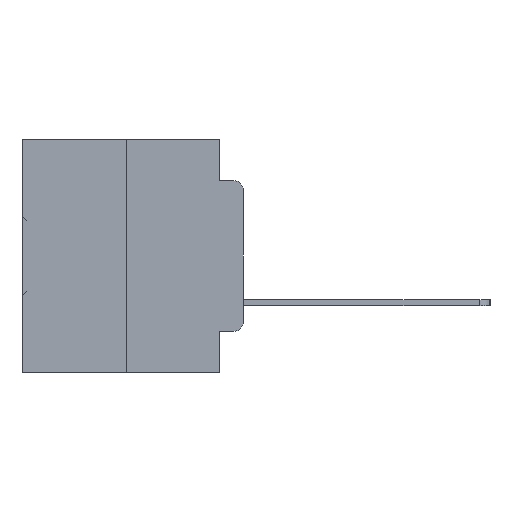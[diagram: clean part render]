
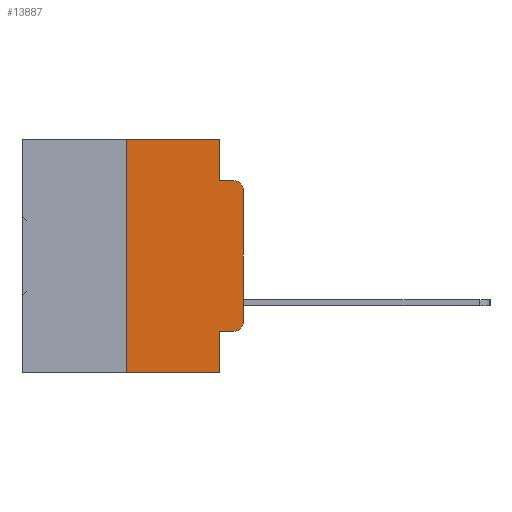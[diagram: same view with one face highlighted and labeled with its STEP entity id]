
A CAD part, left-side view. The second image highlights one B-rep face of the part: STEP entity #13887.
In plain terms, the highlighted planar face has unit normal (-1, 0, 0).
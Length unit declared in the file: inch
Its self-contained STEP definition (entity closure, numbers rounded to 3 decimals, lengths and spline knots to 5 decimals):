
#2 = DIRECTION ( 'NONE',  ( 0., 0., -1. ) ) ;
#71 = CARTESIAN_POINT ( 'NONE',  ( 0., 0.473, 0. ) ) ;
#235 = VERTEX_POINT ( 'NONE', #4766 ) ;
#957 = CARTESIAN_POINT ( 'NONE',  ( 0., 0.473, -0.5 ) ) ;
#1449 = ORIENTED_EDGE ( 'NONE', *, *, #22630, .F. ) ;
#1769 = DIRECTION ( 'NONE',  ( -1., 0., 0. ) ) ;
#2071 = FACE_OUTER_BOUND ( 'NONE', #31093, .T. ) ;
#3737 = CARTESIAN_POINT ( 'NONE',  ( 0., 0.473, 0. ) ) ;
#4766 = CARTESIAN_POINT ( 'NONE',  ( 0., 0., -0.3915 ) ) ;
#5221 = CIRCLE ( 'NONE', #13717, 0.02 ) ;
#5657 = ORIENTED_EDGE ( 'NONE', *, *, #19311, .F. ) ;
#5846 = EDGE_CURVE ( 'NONE', #35466, #235, #33170, .T. ) ;
#6300 = CARTESIAN_POINT ( 'NONE',  ( 0., 0., -0.1085 ) ) ;
#6309 = CARTESIAN_POINT ( 'NONE',  ( 0., 0.25, -0.5 ) ) ;
#6645 = DIRECTION ( 'NONE',  ( 0., 0., -1. ) ) ;
#6834 = CARTESIAN_POINT ( 'NONE',  ( 0., 0.02, -0.1085 ) ) ;
#7012 = VERTEX_POINT ( 'NONE', #32410 ) ;
#7473 = VECTOR ( 'NONE', #2, 39.37008 ) ;
#7770 = EDGE_CURVE ( 'NONE', #29344, #35466, #22301, .T. ) ;
#8345 = ORIENTED_EDGE ( 'NONE', *, *, #15532, .F. ) ;
#8763 = EDGE_CURVE ( 'NONE', #29814, #9407, #18741, .T. ) ;
#9239 = ORIENTED_EDGE ( 'NONE', *, *, #8763, .T. ) ;
#9267 = VECTOR ( 'NONE', #19832, 39.37008 ) ;
#9407 = VERTEX_POINT ( 'NONE', #34750 ) ;
#9705 = EDGE_CURVE ( 'NONE', #29344, #9407, #15171, .T. ) ;
#9732 = DIRECTION ( 'NONE',  ( 0., 0., -1. ) ) ;
#10631 = ORIENTED_EDGE ( 'NONE', *, *, #5846, .T. ) ;
#11118 = AXIS2_PLACEMENT_3D ( 'NONE', #3737, #23708, #6645 ) ;
#12925 = VECTOR ( 'NONE', #28547, 39.37008 ) ;
#12945 = CARTESIAN_POINT ( 'NONE',  ( 0., 0.02, -0.4115 ) ) ;
#13552 = EDGE_CURVE ( 'NONE', #29814, #33952, #13873, .T. ) ;
#13717 = AXIS2_PLACEMENT_3D ( 'NONE', #6834, #26666, #9732 ) ;
#13873 = LINE ( 'NONE', #28134, #20551 ) ;
#13887 = ADVANCED_FACE ( 'NONE', ( #2071 ), #31814, .F. ) ;
#14195 = CARTESIAN_POINT ( 'NONE',  ( 0., 0.051, -0.0885 ) ) ;
#15171 = LINE ( 'NONE', #25613, #7473 ) ;
#15532 = EDGE_CURVE ( 'NONE', #27785, #34125, #20039, .T. ) ;
#16621 = VECTOR ( 'NONE', #19922, 39.37008 ) ;
#17033 = AXIS2_PLACEMENT_3D ( 'NONE', #19036, #1769, #21828 ) ;
#17379 = ORIENTED_EDGE ( 'NONE', *, *, #7770, .T. ) ;
#18741 = LINE ( 'NONE', #957, #25280 ) ;
#19036 = CARTESIAN_POINT ( 'NONE',  ( 0., 0.02, -0.3915 ) ) ;
#19311 = EDGE_CURVE ( 'NONE', #34125, #7012, #24078, .T. ) ;
#19776 = CARTESIAN_POINT ( 'NONE',  ( 0., 0.051, -0.4115 ) ) ;
#19832 = DIRECTION ( 'NONE',  ( 0., 0., -1. ) ) ;
#19922 = DIRECTION ( 'NONE',  ( 0., -1., 0. ) ) ;
#19992 = VERTEX_POINT ( 'NONE', #6300 ) ;
#20039 = LINE ( 'NONE', #33493, #9267 ) ;
#20048 = ORIENTED_EDGE ( 'NONE', *, *, #13552, .F. ) ;
#20539 = LINE ( 'NONE', #71, #12925 ) ;
#20551 = VECTOR ( 'NONE', #25374, 39.37008 ) ;
#20868 = ORIENTED_EDGE ( 'NONE', *, *, #21171, .T. ) ;
#21171 = EDGE_CURVE ( 'NONE', #19992, #7012, #5221, .T. ) ;
#21203 = CARTESIAN_POINT ( 'NONE',  ( 0., 0.051, -0.4115 ) ) ;
#21828 = DIRECTION ( 'NONE',  ( 0., 0., -1. ) ) ;
#22301 = LINE ( 'NONE', #19776, #35993 ) ;
#22630 = EDGE_CURVE ( 'NONE', #33952, #27785, #20539, .T. ) ;
#23708 = DIRECTION ( 'NONE',  ( 1., 0., 0. ) ) ;
#24078 = LINE ( 'NONE', #14195, #16621 ) ;
#24895 = EDGE_CURVE ( 'NONE', #235, #19992, #29827, .T. ) ;
#25280 = VECTOR ( 'NONE', #31970, 39.37008 ) ;
#25374 = DIRECTION ( 'NONE',  ( 0., 0., 1. ) ) ;
#25613 = CARTESIAN_POINT ( 'NONE',  ( 0., 0.051, 0. ) ) ;
#26666 = DIRECTION ( 'NONE',  ( -1., 0., 0. ) ) ;
#27785 = VERTEX_POINT ( 'NONE', #36203 ) ;
#28119 = DIRECTION ( 'NONE',  ( 0., -1., 0. ) ) ;
#28134 = CARTESIAN_POINT ( 'NONE',  ( 0., 0.25, 0. ) ) ;
#28547 = DIRECTION ( 'NONE',  ( 0., -1., 0. ) ) ;
#28994 = VECTOR ( 'NONE', #36110, 39.37008 ) ;
#29332 = CARTESIAN_POINT ( 'NONE',  ( 0., 0.051, -0.0885 ) ) ;
#29344 = VERTEX_POINT ( 'NONE', #21203 ) ;
#29814 = VERTEX_POINT ( 'NONE', #6309 ) ;
#29827 = LINE ( 'NONE', #33376, #28994 ) ;
#31093 = EDGE_LOOP ( 'NONE', ( #32867, #20868, #5657, #8345, #1449, #20048, #9239, #32447, #17379, #10631 ) ) ;
#31814 = PLANE ( 'NONE',  #11118 ) ;
#31970 = DIRECTION ( 'NONE',  ( 0., -1., 0. ) ) ;
#32410 = CARTESIAN_POINT ( 'NONE',  ( 0., 0.02, -0.0885 ) ) ;
#32447 = ORIENTED_EDGE ( 'NONE', *, *, #9705, .F. ) ;
#32867 = ORIENTED_EDGE ( 'NONE', *, *, #24895, .T. ) ;
#33170 = CIRCLE ( 'NONE', #17033, 0.02 ) ;
#33376 = CARTESIAN_POINT ( 'NONE',  ( 0., 0., 0. ) ) ;
#33485 = CARTESIAN_POINT ( 'NONE',  ( 0., 0.25, 0. ) ) ;
#33493 = CARTESIAN_POINT ( 'NONE',  ( 0., 0.051, 0. ) ) ;
#33952 = VERTEX_POINT ( 'NONE', #33485 ) ;
#34125 = VERTEX_POINT ( 'NONE', #29332 ) ;
#34750 = CARTESIAN_POINT ( 'NONE',  ( 0., 0.051, -0.5 ) ) ;
#35466 = VERTEX_POINT ( 'NONE', #12945 ) ;
#35993 = VECTOR ( 'NONE', #28119, 39.37008 ) ;
#36110 = DIRECTION ( 'NONE',  ( 0., 0., 1. ) ) ;
#36203 = CARTESIAN_POINT ( 'NONE',  ( 0., 0.051, 0. ) ) ;
